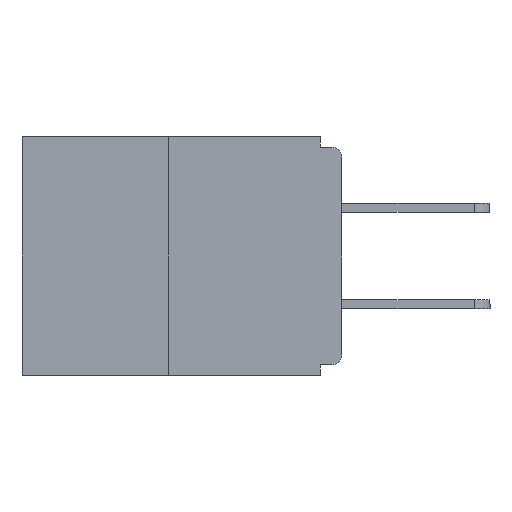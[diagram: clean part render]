
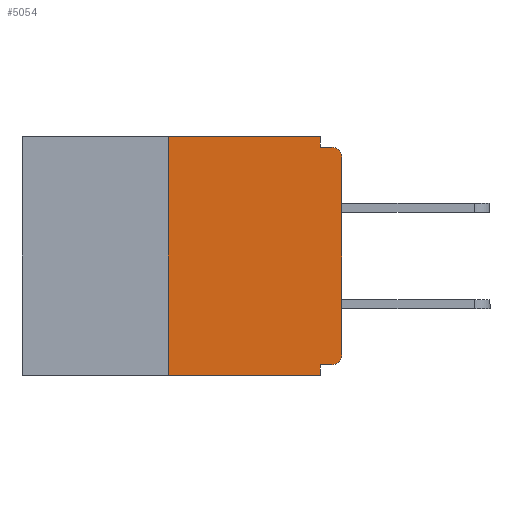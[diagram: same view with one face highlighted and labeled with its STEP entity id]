
A CAD part, left-side view. The second image highlights one B-rep face of the part: STEP entity #5054.
In plain terms, the highlighted planar face has unit normal (-1, 0, 0).
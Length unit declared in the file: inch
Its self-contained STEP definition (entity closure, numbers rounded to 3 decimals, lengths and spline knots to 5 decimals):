
#48 = PLANE ( 'NONE',  #19654 ) ;
#90 = VECTOR ( 'NONE', #25123, 39.37008 ) ;
#137 = CARTESIAN_POINT ( 'NONE',  ( 0., 0.46, 0. ) ) ;
#150 = FACE_OUTER_BOUND ( 'NONE', #23604, .T. ) ;
#183 = EDGE_CURVE ( 'NONE', #22243, #17790, #19531, .T. ) ;
#314 = CIRCLE ( 'NONE', #25437, 0.015 ) ;
#316 = ORIENTED_EDGE ( 'NONE', *, *, #27093, .T. ) ;
#1410 = CARTESIAN_POINT ( 'NONE',  ( 0., 0.015, -0.015 ) ) ;
#1582 = ORIENTED_EDGE ( 'NONE', *, *, #10902, .F. ) ;
#1722 = DIRECTION ( 'NONE',  ( 0., -1., 0. ) ) ;
#2010 = CARTESIAN_POINT ( 'NONE',  ( 0., 0.031, 0. ) ) ;
#2302 = LINE ( 'NONE', #9579, #24891 ) ;
#3144 = VERTEX_POINT ( 'NONE', #13383 ) ;
#3704 = LINE ( 'NONE', #14480, #90 ) ;
#4350 = VERTEX_POINT ( 'NONE', #6708 ) ;
#4646 = ORIENTED_EDGE ( 'NONE', *, *, #7818, .F. ) ;
#4767 = CARTESIAN_POINT ( 'NONE',  ( 0., 0.031, -0.328 ) ) ;
#5054 = ADVANCED_FACE ( 'NONE', ( #150 ), #48, .F. ) ;
#5261 = CARTESIAN_POINT ( 'NONE',  ( 0., 0., -0.313 ) ) ;
#5981 = DIRECTION ( 'NONE',  ( 0., 0., -1. ) ) ;
#5983 = EDGE_CURVE ( 'NONE', #11422, #11804, #19088, .T. ) ;
#6028 = DIRECTION ( 'NONE',  ( 1., 0., 0. ) ) ;
#6691 = EDGE_CURVE ( 'NONE', #4350, #23245, #3704, .T. ) ;
#6708 = CARTESIAN_POINT ( 'NONE',  ( 0., 0.25, -0.343 ) ) ;
#6782 = LINE ( 'NONE', #11549, #12003 ) ;
#6982 = CARTESIAN_POINT ( 'NONE',  ( 0., 0.46, 0. ) ) ;
#7492 = ORIENTED_EDGE ( 'NONE', *, *, #183, .F. ) ;
#7669 = VECTOR ( 'NONE', #21438, 39.37008 ) ;
#7775 = ORIENTED_EDGE ( 'NONE', *, *, #26560, .F. ) ;
#7818 = EDGE_CURVE ( 'NONE', #15381, #3144, #6782, .T. ) ;
#9374 = DIRECTION ( 'NONE',  ( 0., 0., -1. ) ) ;
#9579 = CARTESIAN_POINT ( 'NONE',  ( 0., 0., -0.328 ) ) ;
#9769 = VECTOR ( 'NONE', #1722, 39.37008 ) ;
#10504 = DIRECTION ( 'NONE',  ( 0., 0., -1. ) ) ;
#10902 = EDGE_CURVE ( 'NONE', #23245, #16873, #14521, .T. ) ;
#11422 = VERTEX_POINT ( 'NONE', #5261 ) ;
#11549 = CARTESIAN_POINT ( 'NONE',  ( 0., 0.031, -0.343 ) ) ;
#11804 = VERTEX_POINT ( 'NONE', #24335 ) ;
#11814 = EDGE_CURVE ( 'NONE', #12726, #15381, #2302, .T. ) ;
#12003 = VECTOR ( 'NONE', #19598, 39.37008 ) ;
#12726 = VERTEX_POINT ( 'NONE', #13560 ) ;
#12972 = DIRECTION ( 'NONE',  ( 0., -1., 0. ) ) ;
#13383 = CARTESIAN_POINT ( 'NONE',  ( 0., 0.031, -0.343 ) ) ;
#13395 = CARTESIAN_POINT ( 'NONE',  ( 0., 0., -0.015 ) ) ;
#13560 = CARTESIAN_POINT ( 'NONE',  ( 0., 0.015, -0.328 ) ) ;
#14279 = EDGE_CURVE ( 'NONE', #12726, #11422, #314, .T. ) ;
#14480 = CARTESIAN_POINT ( 'NONE',  ( 0., 0.25, 0. ) ) ;
#14521 = LINE ( 'NONE', #6982, #24947 ) ;
#14693 = LINE ( 'NONE', #17074, #15706 ) ;
#15049 = EDGE_CURVE ( 'NONE', #4350, #3144, #14693, .T. ) ;
#15381 = VERTEX_POINT ( 'NONE', #4767 ) ;
#15706 = VECTOR ( 'NONE', #12972, 39.37008 ) ;
#16226 = ORIENTED_EDGE ( 'NONE', *, *, #5983, .T. ) ;
#16436 = DIRECTION ( 'NONE',  ( -1., 0., 0. ) ) ;
#16472 = CIRCLE ( 'NONE', #21000, 0.015 ) ;
#16566 = DIRECTION ( 'NONE',  ( 0., 0., -1. ) ) ;
#16638 = CARTESIAN_POINT ( 'NONE',  ( 0., 0.25, 0. ) ) ;
#16873 = VERTEX_POINT ( 'NONE', #2010 ) ;
#17074 = CARTESIAN_POINT ( 'NONE',  ( 0., 0.46, -0.343 ) ) ;
#17492 = CARTESIAN_POINT ( 'NONE',  ( 0., 0., 0. ) ) ;
#17764 = LINE ( 'NONE', #21860, #20050 ) ;
#17790 = VERTEX_POINT ( 'NONE', #1410 ) ;
#18036 = DIRECTION ( 'NONE',  ( 0., 1., 0. ) ) ;
#18505 = ORIENTED_EDGE ( 'NONE', *, *, #15049, .T. ) ;
#18569 = CARTESIAN_POINT ( 'NONE',  ( 0., 0.015, -0.313 ) ) ;
#19088 = LINE ( 'NONE', #17492, #7669 ) ;
#19531 = LINE ( 'NONE', #13395, #9769 ) ;
#19598 = DIRECTION ( 'NONE',  ( 0., 0., -1. ) ) ;
#19654 = AXIS2_PLACEMENT_3D ( 'NONE', #137, #6028, #16566 ) ;
#20050 = VECTOR ( 'NONE', #9374, 39.37008 ) ;
#21000 = AXIS2_PLACEMENT_3D ( 'NONE', #25088, #25195, #10504 ) ;
#21438 = DIRECTION ( 'NONE',  ( 0., 0., 1. ) ) ;
#21860 = CARTESIAN_POINT ( 'NONE',  ( 0., 0.031, 0. ) ) ;
#22131 = ORIENTED_EDGE ( 'NONE', *, *, #6691, .F. ) ;
#22243 = VERTEX_POINT ( 'NONE', #23096 ) ;
#23096 = CARTESIAN_POINT ( 'NONE',  ( 0., 0.031, -0.015 ) ) ;
#23245 = VERTEX_POINT ( 'NONE', #16638 ) ;
#23388 = ORIENTED_EDGE ( 'NONE', *, *, #11814, .F. ) ;
#23604 = EDGE_LOOP ( 'NONE', ( #1582, #22131, #18505, #4646, #23388, #23969, #16226, #316, #7492, #7775 ) ) ;
#23969 = ORIENTED_EDGE ( 'NONE', *, *, #14279, .T. ) ;
#24335 = CARTESIAN_POINT ( 'NONE',  ( 0., 0., -0.03 ) ) ;
#24891 = VECTOR ( 'NONE', #18036, 39.37008 ) ;
#24947 = VECTOR ( 'NONE', #25616, 39.37008 ) ;
#25088 = CARTESIAN_POINT ( 'NONE',  ( 0., 0.015, -0.03 ) ) ;
#25123 = DIRECTION ( 'NONE',  ( 0., 0., 1. ) ) ;
#25195 = DIRECTION ( 'NONE',  ( -1., 0., 0. ) ) ;
#25437 = AXIS2_PLACEMENT_3D ( 'NONE', #18569, #16436, #5981 ) ;
#25616 = DIRECTION ( 'NONE',  ( 0., -1., 0. ) ) ;
#26560 = EDGE_CURVE ( 'NONE', #16873, #22243, #17764, .T. ) ;
#27093 = EDGE_CURVE ( 'NONE', #11804, #17790, #16472, .T. ) ;
